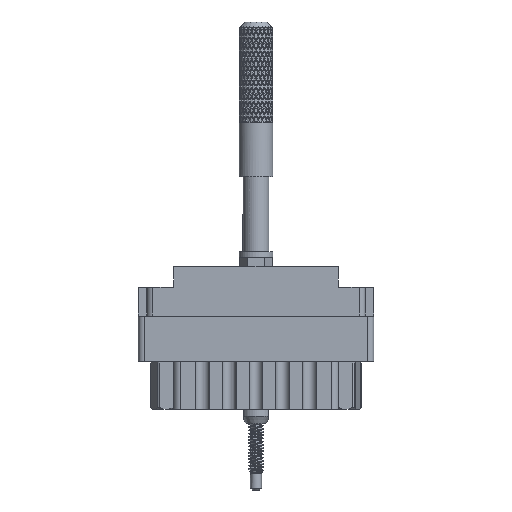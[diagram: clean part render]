
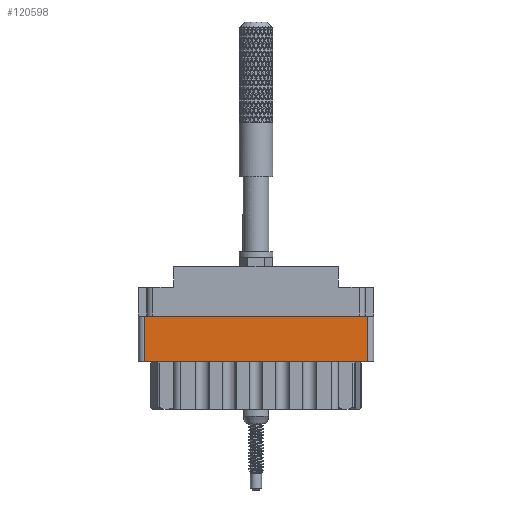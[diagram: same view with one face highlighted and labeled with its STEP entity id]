
A CAD part, front view. The second image highlights one B-rep face of the part: STEP entity #120598.
In plain terms, the highlighted planar face has unit normal (0, -1, 0).
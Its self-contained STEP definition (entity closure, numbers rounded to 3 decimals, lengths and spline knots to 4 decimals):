
#1544 = AXIS2_PLACEMENT_3D ( 'NONE', #33455, #15858, #120874 ) ;
#2532 = CARTESIAN_POINT ( 'NONE',  ( -0.624, -0.343, -0.798 ) ) ;
#3440 = PLANE ( 'NONE',  #1544 ) ;
#15858 = DIRECTION ( 'NONE',  ( 0., -1., 0. ) ) ;
#22416 = FACE_OUTER_BOUND ( 'NONE', #119570, .T. ) ;
#27225 = VERTEX_POINT ( 'NONE', #106019 ) ;
#29231 = ORIENTED_EDGE ( 'NONE', *, *, #177722, .F. ) ;
#30647 = CARTESIAN_POINT ( 'NONE',  ( -0.624, -0.343, -0.529 ) ) ;
#33455 = CARTESIAN_POINT ( 'NONE',  ( -0.656, -0.343, -0.798 ) ) ;
#38390 = EDGE_CURVE ( 'NONE', #27225, #46667, #47413, .T. ) ;
#39813 = DIRECTION ( 'NONE',  ( 1., 0., 0. ) ) ;
#41010 = ORIENTED_EDGE ( 'NONE', *, *, #84533, .F. ) ;
#41323 = VECTOR ( 'NONE', #103351, 39.3701 ) ;
#46667 = VERTEX_POINT ( 'NONE', #30647 ) ;
#47413 = LINE ( 'NONE', #2532, #94024 ) ;
#49546 = CARTESIAN_POINT ( 'NONE',  ( 0.624, -0.343, -0.529 ) ) ;
#56112 = CARTESIAN_POINT ( 'NONE',  ( 0.624, -0.343, -0.277 ) ) ;
#74695 = ORIENTED_EDGE ( 'NONE', *, *, #168507, .T. ) ;
#76343 = LINE ( 'NONE', #88352, #41323 ) ;
#84533 = EDGE_CURVE ( 'NONE', #27225, #176165, #139932, .T. ) ;
#88352 = CARTESIAN_POINT ( 'NONE',  ( 0., -0.343, -0.529 ) ) ;
#94024 = VECTOR ( 'NONE', #94528, 39.3701 ) ;
#94528 = DIRECTION ( 'NONE',  ( 0., 0., -1. ) ) ;
#99224 = CARTESIAN_POINT ( 'NONE',  ( 0., -0.343, -0.277 ) ) ;
#101866 = CARTESIAN_POINT ( 'NONE',  ( 0.624, -0.343, -0.798 ) ) ;
#103351 = DIRECTION ( 'NONE',  ( -1., 0., 0. ) ) ;
#106019 = CARTESIAN_POINT ( 'NONE',  ( -0.624, -0.343, -0.277 ) ) ;
#119570 = EDGE_LOOP ( 'NONE', ( #41010, #172497, #29231, #74695 ) ) ;
#120598 = ADVANCED_FACE ( 'NONE', ( #22416 ), #3440, .T. ) ;
#120874 = DIRECTION ( 'NONE',  ( 0., 0., -1. ) ) ;
#139932 = LINE ( 'NONE', #99224, #188982 ) ;
#158455 = VERTEX_POINT ( 'NONE', #49546 ) ;
#168507 = EDGE_CURVE ( 'NONE', #158455, #176165, #171137, .T. ) ;
#171137 = LINE ( 'NONE', #101866, #185218 ) ;
#172497 = ORIENTED_EDGE ( 'NONE', *, *, #38390, .T. ) ;
#176165 = VERTEX_POINT ( 'NONE', #56112 ) ;
#177722 = EDGE_CURVE ( 'NONE', #158455, #46667, #76343, .T. ) ;
#185218 = VECTOR ( 'NONE', #191696, 39.3701 ) ;
#188982 = VECTOR ( 'NONE', #39813, 39.3701 ) ;
#191696 = DIRECTION ( 'NONE',  ( 0., 0., 1. ) ) ;
